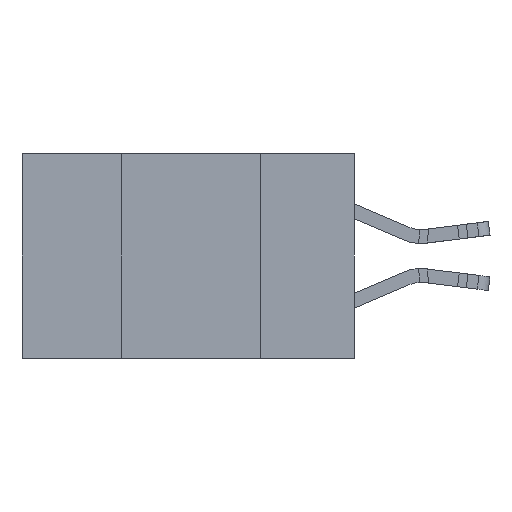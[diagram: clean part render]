
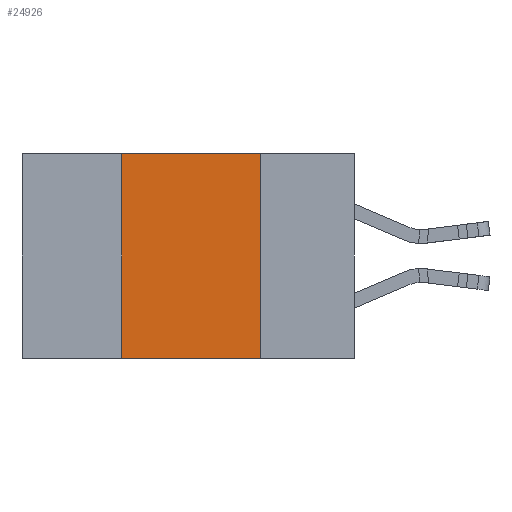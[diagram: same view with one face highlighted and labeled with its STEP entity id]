
A CAD part, left-side view. The second image highlights one B-rep face of the part: STEP entity #24926.
In plain terms, the highlighted planar face has unit normal (-1, 0, 0).
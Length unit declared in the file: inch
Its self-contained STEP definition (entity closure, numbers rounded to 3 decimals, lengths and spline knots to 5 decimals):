
#26 = VERTEX_POINT ( 'NONE', #19251 ) ;
#55 = VECTOR ( 'NONE', #13306, 39.37008 ) ;
#749 = ORIENTED_EDGE ( 'NONE', *, *, #27296, .T. ) ;
#2147 = EDGE_CURVE ( 'NONE', #3605, #26, #26778, .T. ) ;
#2333 = FACE_OUTER_BOUND ( 'NONE', #15675, .T. ) ;
#2470 = DIRECTION ( 'NONE',  ( 0., 0., -1. ) ) ;
#3329 = LINE ( 'NONE', #24654, #14145 ) ;
#3605 = VERTEX_POINT ( 'NONE', #3960 ) ;
#3960 = CARTESIAN_POINT ( 'NONE',  ( 0., 0.17, 0. ) ) ;
#4554 = PLANE ( 'NONE',  #27201 ) ;
#7272 = LINE ( 'NONE', #16054, #9984 ) ;
#9984 = VECTOR ( 'NONE', #13552, 39.37008 ) ;
#11264 = CARTESIAN_POINT ( 'NONE',  ( 0., 0.42, 0. ) ) ;
#13306 = DIRECTION ( 'NONE',  ( 0., 0., -1. ) ) ;
#13552 = DIRECTION ( 'NONE',  ( 0., -1., 0. ) ) ;
#13562 = DIRECTION ( 'NONE',  ( 1., 0., 0. ) ) ;
#14145 = VECTOR ( 'NONE', #16148, 39.37008 ) ;
#15675 = EDGE_LOOP ( 'NONE', ( #24867, #27293, #24204, #749 ) ) ;
#16054 = CARTESIAN_POINT ( 'NONE',  ( 0., 0.6, -0.37 ) ) ;
#16148 = DIRECTION ( 'NONE',  ( 0., -1., 0. ) ) ;
#16966 = CARTESIAN_POINT ( 'NONE',  ( 0., 0.6, 0. ) ) ;
#18701 = LINE ( 'NONE', #27345, #19496 ) ;
#19251 = CARTESIAN_POINT ( 'NONE',  ( 0., 0.17, -0.37 ) ) ;
#19496 = VECTOR ( 'NONE', #24834, 39.37008 ) ;
#19957 = EDGE_CURVE ( 'NONE', #24619, #3605, #3329, .T. ) ;
#21511 = EDGE_CURVE ( 'NONE', #25417, #24619, #18701, .T. ) ;
#23442 = CARTESIAN_POINT ( 'NONE',  ( 0., 0.42, -0.37 ) ) ;
#24204 = ORIENTED_EDGE ( 'NONE', *, *, #21511, .F. ) ;
#24619 = VERTEX_POINT ( 'NONE', #11264 ) ;
#24654 = CARTESIAN_POINT ( 'NONE',  ( 0., 0.6, 0. ) ) ;
#24834 = DIRECTION ( 'NONE',  ( 0., 0., 1. ) ) ;
#24867 = ORIENTED_EDGE ( 'NONE', *, *, #2147, .F. ) ;
#24926 = ADVANCED_FACE ( 'NONE', ( #2333 ), #4554, .F. ) ;
#25417 = VERTEX_POINT ( 'NONE', #23442 ) ;
#26778 = LINE ( 'NONE', #26915, #55 ) ;
#26915 = CARTESIAN_POINT ( 'NONE',  ( 0., 0.17, -0.37 ) ) ;
#27201 = AXIS2_PLACEMENT_3D ( 'NONE', #16966, #13562, #2470 ) ;
#27293 = ORIENTED_EDGE ( 'NONE', *, *, #19957, .F. ) ;
#27296 = EDGE_CURVE ( 'NONE', #25417, #26, #7272, .T. ) ;
#27345 = CARTESIAN_POINT ( 'NONE',  ( 0., 0.42, -0.37 ) ) ;
